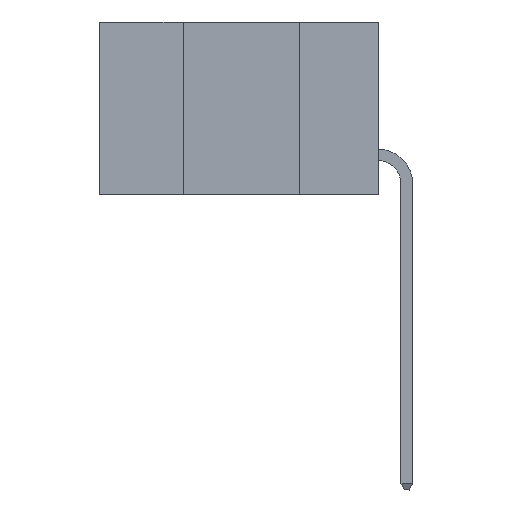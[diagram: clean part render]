
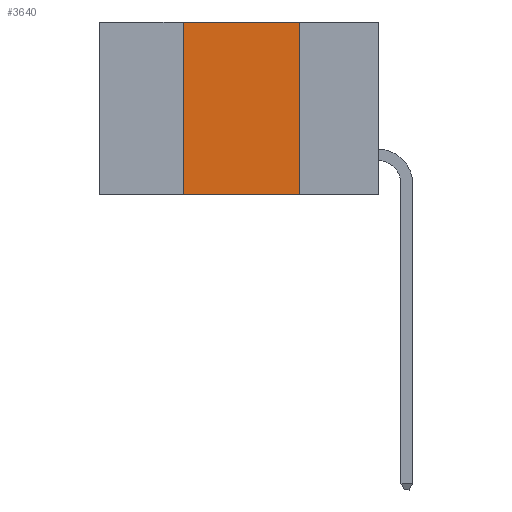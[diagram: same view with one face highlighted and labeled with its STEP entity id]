
A CAD part, left-side view. The second image highlights one B-rep face of the part: STEP entity #3640.
In plain terms, the highlighted planar face has unit normal (-1, 0, 0).
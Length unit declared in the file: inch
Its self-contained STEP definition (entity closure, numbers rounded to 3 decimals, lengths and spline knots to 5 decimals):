
#195 = LINE ( 'NONE', #14709, #14016 ) ;
#2741 = EDGE_CURVE ( 'NONE', #8485, #9365, #13295, .T. ) ;
#2854 = VERTEX_POINT ( 'NONE', #11255 ) ;
#2876 = DIRECTION ( 'NONE',  ( 0., 0., -1. ) ) ;
#2879 = CARTESIAN_POINT ( 'NONE',  ( 0., 0.17, 0. ) ) ;
#2979 = ORIENTED_EDGE ( 'NONE', *, *, #11481, .T. ) ;
#3268 = ORIENTED_EDGE ( 'NONE', *, *, #2741, .F. ) ;
#3640 = ADVANCED_FACE ( 'NONE', ( #18039 ), #10900, .F. ) ;
#3795 = DIRECTION ( 'NONE',  ( 1., 0., 0. ) ) ;
#3924 = DIRECTION ( 'NONE',  ( 0., 0., -1. ) ) ;
#4741 = LINE ( 'NONE', #8502, #13006 ) ;
#5090 = CARTESIAN_POINT ( 'NONE',  ( 0., 0.6, 0. ) ) ;
#5856 = LINE ( 'NONE', #11781, #7188 ) ;
#6285 = DIRECTION ( 'NONE',  ( 0., -1., 0. ) ) ;
#7051 = EDGE_LOOP ( 'NONE', ( #7884, #3268, #17395, #2979 ) ) ;
#7188 = VECTOR ( 'NONE', #6285, 39.37008 ) ;
#7884 = ORIENTED_EDGE ( 'NONE', *, *, #11312, .F. ) ;
#8306 = CARTESIAN_POINT ( 'NONE',  ( 0., 0.17, -0.37 ) ) ;
#8485 = VERTEX_POINT ( 'NONE', #14229 ) ;
#8502 = CARTESIAN_POINT ( 'NONE',  ( 0., 0.17, 0. ) ) ;
#9365 = VERTEX_POINT ( 'NONE', #2879 ) ;
#9945 = VECTOR ( 'NONE', #13761, 39.37008 ) ;
#10900 = PLANE ( 'NONE',  #13120 ) ;
#11255 = CARTESIAN_POINT ( 'NONE',  ( 0., 0.42, -0.37 ) ) ;
#11312 = EDGE_CURVE ( 'NONE', #9365, #12040, #4741, .T. ) ;
#11481 = EDGE_CURVE ( 'NONE', #2854, #12040, #5856, .T. ) ;
#11781 = CARTESIAN_POINT ( 'NONE',  ( 0., 0.6, -0.37 ) ) ;
#12040 = VERTEX_POINT ( 'NONE', #8306 ) ;
#13006 = VECTOR ( 'NONE', #2876, 39.37008 ) ;
#13120 = AXIS2_PLACEMENT_3D ( 'NONE', #15280, #3795, #3924 ) ;
#13295 = LINE ( 'NONE', #5090, #9945 ) ;
#13455 = DIRECTION ( 'NONE',  ( 0., 0., 1. ) ) ;
#13761 = DIRECTION ( 'NONE',  ( 0., -1., 0. ) ) ;
#14016 = VECTOR ( 'NONE', #13455, 39.37008 ) ;
#14229 = CARTESIAN_POINT ( 'NONE',  ( 0., 0.42, 0. ) ) ;
#14709 = CARTESIAN_POINT ( 'NONE',  ( 0., 0.42, 0. ) ) ;
#15070 = EDGE_CURVE ( 'NONE', #2854, #8485, #195, .T. ) ;
#15280 = CARTESIAN_POINT ( 'NONE',  ( 0., 0.6, 0. ) ) ;
#17395 = ORIENTED_EDGE ( 'NONE', *, *, #15070, .F. ) ;
#18039 = FACE_OUTER_BOUND ( 'NONE', #7051, .T. ) ;
